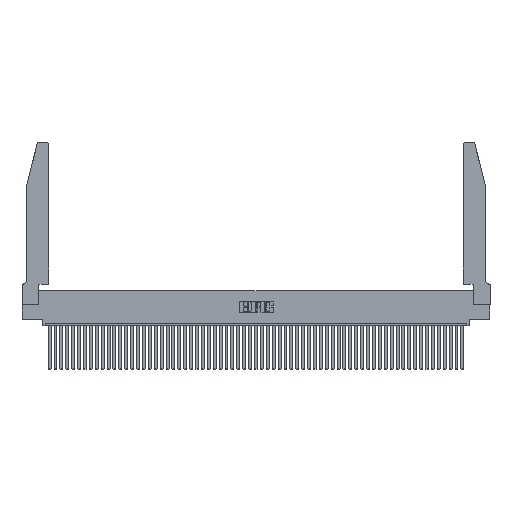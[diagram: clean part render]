
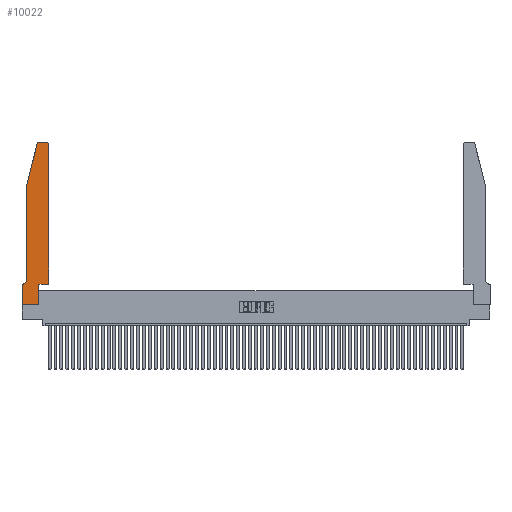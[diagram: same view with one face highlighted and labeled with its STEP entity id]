
A CAD part, top view. The second image highlights one B-rep face of the part: STEP entity #10022.
In plain terms, the highlighted planar face has unit normal (0, 0, 1).
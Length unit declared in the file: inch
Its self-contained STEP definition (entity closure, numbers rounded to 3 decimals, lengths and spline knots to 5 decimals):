
#2259 = VECTOR ( 'NONE', #46306, 39.37008 ) ;
#2597 = VECTOR ( 'NONE', #37280, 39.37008 ) ;
#3947 = LINE ( 'NONE', #4296, #2597 ) ;
#4296 = CARTESIAN_POINT ( 'NONE',  ( 0.2605, 2.75, 0.37 ) ) ;
#4522 = CIRCLE ( 'NONE', #50468, 0.03 ) ;
#5539 = EDGE_CURVE ( 'NONE', #24608, #17644, #36064, .T. ) ;
#6141 = CARTESIAN_POINT ( 'NONE',  ( 0., 0.35, 0.37 ) ) ;
#6826 = EDGE_CURVE ( 'NONE', #27087, #28478, #11643, .T. ) ;
#6952 = CARTESIAN_POINT ( 'NONE',  ( 0.4505, 2.72, 0.37 ) ) ;
#7484 = CARTESIAN_POINT ( 'NONE',  ( 0.4505, 0.35, 0.37 ) ) ;
#8703 = ORIENTED_EDGE ( 'NONE', *, *, #26186, .T. ) ;
#8986 = CARTESIAN_POINT ( 'NONE',  ( 0.0755, 0.35, 0.37 ) ) ;
#10022 = ADVANCED_FACE ( 'NONE', ( #40808 ), #39815, .T. ) ;
#10334 = DIRECTION ( 'NONE',  ( 0., 0., 1. ) ) ;
#10371 = CARTESIAN_POINT ( 'NONE',  ( 0., 0.35, 0.37 ) ) ;
#11054 = CARTESIAN_POINT ( 'NONE',  ( 0.0055, 0.42, 0.37 ) ) ;
#11321 = VERTEX_POINT ( 'NONE', #28347 ) ;
#11643 = CIRCLE ( 'NONE', #37365, 0.03 ) ;
#11760 = DIRECTION ( 'NONE',  ( 1., 0., 0. ) ) ;
#11937 = CARTESIAN_POINT ( 'NONE',  ( 0.4205, 2.72, 0.37 ) ) ;
#12462 = EDGE_LOOP ( 'NONE', ( #50863, #45028, #17877, #51543, #27159, #37478, #18886, #22598, #40220, #13830, #24597, #8703 ) ) ;
#13830 = ORIENTED_EDGE ( 'NONE', *, *, #26937, .T. ) ;
#14268 = CARTESIAN_POINT ( 'NONE',  ( 0.0755, 2., 0.37 ) ) ;
#15645 = LINE ( 'NONE', #24519, #26009 ) ;
#16742 = CARTESIAN_POINT ( 'NONE',  ( 0.4505, 0.35, 0.37 ) ) ;
#16775 = DIRECTION ( 'NONE',  ( 0., -1., 0. ) ) ;
#17533 = VERTEX_POINT ( 'NONE', #6952 ) ;
#17627 = CARTESIAN_POINT ( 'NONE',  ( 0., 0., 0.37 ) ) ;
#17644 = VERTEX_POINT ( 'NONE', #38307 ) ;
#17877 = ORIENTED_EDGE ( 'NONE', *, *, #28390, .T. ) ;
#18886 = ORIENTED_EDGE ( 'NONE', *, *, #44078, .T. ) ;
#19045 = AXIS2_PLACEMENT_3D ( 'NONE', #11054, #22971, #44174 ) ;
#20561 = EDGE_CURVE ( 'NONE', #25878, #17533, #15645, .T. ) ;
#20709 = DIRECTION ( 'NONE',  ( 1., 0., 0. ) ) ;
#20751 = LINE ( 'NONE', #17627, #2259 ) ;
#21325 = AXIS2_PLACEMENT_3D ( 'NONE', #6141, #10334, #22999 ) ;
#22598 = ORIENTED_EDGE ( 'NONE', *, *, #25603, .T. ) ;
#22971 = DIRECTION ( 'NONE',  ( 0., 0., -1. ) ) ;
#22999 = DIRECTION ( 'NONE',  ( 1., 0., 0. ) ) ;
#24519 = CARTESIAN_POINT ( 'NONE',  ( 0.4505, 0.35, 0.37 ) ) ;
#24597 = ORIENTED_EDGE ( 'NONE', *, *, #20561, .T. ) ;
#24608 = VERTEX_POINT ( 'NONE', #49225 ) ;
#24956 = VECTOR ( 'NONE', #26646, 39.37008 ) ;
#25603 = EDGE_CURVE ( 'NONE', #51602, #24608, #49793, .T. ) ;
#25878 = VERTEX_POINT ( 'NONE', #16742 ) ;
#26009 = VECTOR ( 'NONE', #39042, 39.37008 ) ;
#26186 = EDGE_CURVE ( 'NONE', #17533, #46408, #4522, .T. ) ;
#26498 = CIRCLE ( 'NONE', #19045, 0.07 ) ;
#26540 = LINE ( 'NONE', #33409, #27885 ) ;
#26646 = DIRECTION ( 'NONE',  ( 0., 1., 0. ) ) ;
#26937 = EDGE_CURVE ( 'NONE', #17644, #25878, #49025, .T. ) ;
#27087 = VERTEX_POINT ( 'NONE', #27528 ) ;
#27159 = ORIENTED_EDGE ( 'NONE', *, *, #50331, .T. ) ;
#27528 = CARTESIAN_POINT ( 'NONE',  ( 0.284, 2.75, 0.37 ) ) ;
#27885 = VECTOR ( 'NONE', #16775, 39.37008 ) ;
#28347 = CARTESIAN_POINT ( 'NONE',  ( 0.0055, 0.35, 0.37 ) ) ;
#28390 = EDGE_CURVE ( 'NONE', #28478, #30871, #47495, .T. ) ;
#28436 = CARTESIAN_POINT ( 'NONE',  ( 0.0755, 0.42, 0.37 ) ) ;
#28478 = VERTEX_POINT ( 'NONE', #48754 ) ;
#29661 = DIRECTION ( 'NONE',  ( -1., 0., 0. ) ) ;
#30428 = CARTESIAN_POINT ( 'NONE',  ( 0.4205, 2.75, 0.37 ) ) ;
#30871 = VERTEX_POINT ( 'NONE', #14268 ) ;
#32638 = DIRECTION ( 'NONE',  ( 1., 0., 0. ) ) ;
#33409 = CARTESIAN_POINT ( 'NONE',  ( 0.0755, 2., 0.37 ) ) ;
#34929 = CARTESIAN_POINT ( 'NONE',  ( 0.0755, 2., 0.37 ) ) ;
#36064 = LINE ( 'NONE', #44015, #24956 ) ;
#37280 = DIRECTION ( 'NONE',  ( -1., 0., 0. ) ) ;
#37365 = AXIS2_PLACEMENT_3D ( 'NONE', #49203, #38301, #48346 ) ;
#37433 = EDGE_CURVE ( 'NONE', #30871, #50473, #26540, .T. ) ;
#37478 = ORIENTED_EDGE ( 'NONE', *, *, #45224, .T. ) ;
#38301 = DIRECTION ( 'NONE',  ( 0., 0., 1. ) ) ;
#38307 = CARTESIAN_POINT ( 'NONE',  ( 0.2865, 0.35, 0.37 ) ) ;
#39042 = DIRECTION ( 'NONE',  ( 0., 1., 0. ) ) ;
#39815 = PLANE ( 'NONE',  #21325 ) ;
#40220 = ORIENTED_EDGE ( 'NONE', *, *, #5539, .T. ) ;
#40588 = LINE ( 'NONE', #8986, #42469 ) ;
#40808 = FACE_OUTER_BOUND ( 'NONE', #12462, .T. ) ;
#41938 = VECTOR ( 'NONE', #11760, 39.37008 ) ;
#42469 = VECTOR ( 'NONE', #29661, 39.37008 ) ;
#43581 = DIRECTION ( 'NONE',  ( -0.239, -0.971, 0. ) ) ;
#44015 = CARTESIAN_POINT ( 'NONE',  ( 0.2865, 0.35, 0.37 ) ) ;
#44078 = EDGE_CURVE ( 'NONE', #49775, #51602, #20751, .T. ) ;
#44174 = DIRECTION ( 'NONE',  ( -1., 0., 0. ) ) ;
#45028 = ORIENTED_EDGE ( 'NONE', *, *, #6826, .T. ) ;
#45224 = EDGE_CURVE ( 'NONE', #11321, #49775, #40588, .T. ) ;
#46306 = DIRECTION ( 'NONE',  ( 0., -1., 0. ) ) ;
#46348 = VECTOR ( 'NONE', #20709, 39.37008 ) ;
#46408 = VERTEX_POINT ( 'NONE', #30428 ) ;
#47495 = LINE ( 'NONE', #34929, #52771 ) ;
#47977 = CARTESIAN_POINT ( 'NONE',  ( 0., 0., 0.37 ) ) ;
#48346 = DIRECTION ( 'NONE',  ( 1., 0., 0. ) ) ;
#48754 = CARTESIAN_POINT ( 'NONE',  ( 0.25487, 2.72718, 0.37 ) ) ;
#49025 = LINE ( 'NONE', #7484, #46348 ) ;
#49203 = CARTESIAN_POINT ( 'NONE',  ( 0.284, 2.72, 0.37 ) ) ;
#49225 = CARTESIAN_POINT ( 'NONE',  ( 0.2865, 0., 0.37 ) ) ;
#49226 = CARTESIAN_POINT ( 'NONE',  ( 0., 0., 0.37 ) ) ;
#49775 = VERTEX_POINT ( 'NONE', #10371 ) ;
#49793 = LINE ( 'NONE', #49226, #41938 ) ;
#50331 = EDGE_CURVE ( 'NONE', #50473, #11321, #26498, .T. ) ;
#50468 = AXIS2_PLACEMENT_3D ( 'NONE', #11937, #53268, #32638 ) ;
#50473 = VERTEX_POINT ( 'NONE', #28436 ) ;
#50863 = ORIENTED_EDGE ( 'NONE', *, *, #53246, .T. ) ;
#51543 = ORIENTED_EDGE ( 'NONE', *, *, #37433, .T. ) ;
#51602 = VERTEX_POINT ( 'NONE', #47977 ) ;
#52771 = VECTOR ( 'NONE', #43581, 39.37008 ) ;
#53246 = EDGE_CURVE ( 'NONE', #46408, #27087, #3947, .T. ) ;
#53268 = DIRECTION ( 'NONE',  ( 0., 0., 1. ) ) ;
